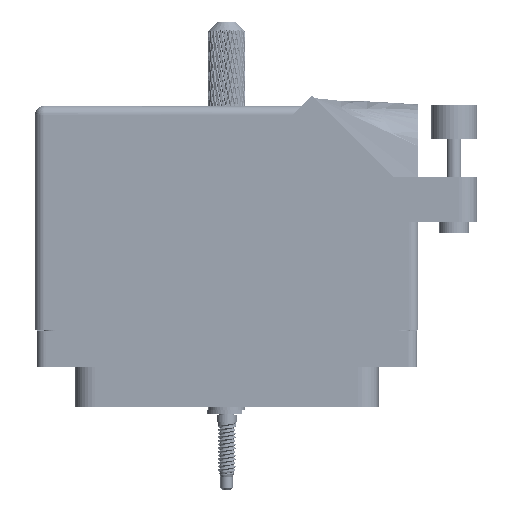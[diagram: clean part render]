
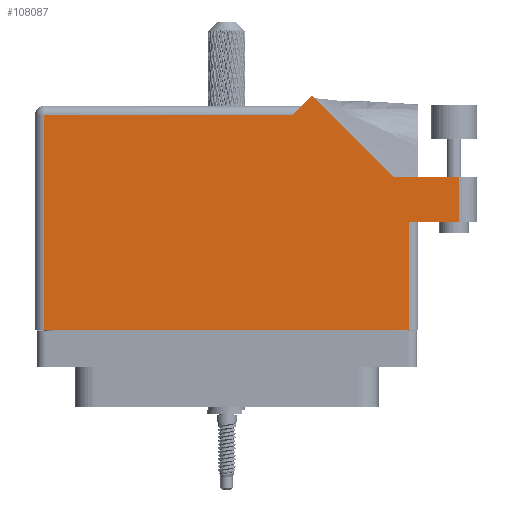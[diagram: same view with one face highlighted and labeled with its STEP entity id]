
A CAD part, front view. The second image highlights one B-rep face of the part: STEP entity #108087.
In plain terms, the highlighted face is planar.
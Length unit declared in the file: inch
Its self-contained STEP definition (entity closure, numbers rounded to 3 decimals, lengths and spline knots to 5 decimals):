
#319 = CARTESIAN_POINT ( 'NONE',  ( -1.306, 1.368, 0.455 ) ) ;
#4055 = ORIENTED_EDGE ( 'NONE', *, *, #53779, .T. ) ;
#4929 = DIRECTION ( 'NONE',  ( 0., 1., 0. ) ) ;
#6549 = ORIENTED_EDGE ( 'NONE', *, *, #40365, .T. ) ;
#8593 = VERTEX_POINT ( 'NONE', #75988 ) ;
#8964 = LINE ( 'NONE', #59721, #91401 ) ;
#10698 = VECTOR ( 'NONE', #41146, 39.37008 ) ;
#11083 = VERTEX_POINT ( 'NONE', #98812 ) ;
#12020 = ORIENTED_EDGE ( 'NONE', *, *, #70977, .T. ) ;
#14296 = LINE ( 'NONE', #103836, #85065 ) ;
#14906 = LINE ( 'NONE', #58714, #114394 ) ;
#15267 = DIRECTION ( 'NONE',  ( 0., -1., 0. ) ) ;
#15478 = VERTEX_POINT ( 'NONE', #91590 ) ;
#21665 = CARTESIAN_POINT ( 'NONE',  ( 1.14042, 0.944, 0.455 ) ) ;
#21743 = CARTESIAN_POINT ( 'NONE',  ( -1.306, 1.43, 0.455 ) ) ;
#21824 = LINE ( 'NONE', #57340, #115629 ) ;
#22697 = ORIENTED_EDGE ( 'NONE', *, *, #76236, .T. ) ;
#24972 = ORIENTED_EDGE ( 'NONE', *, *, #84708, .T. ) ;
#30084 = PLANE ( 'NONE',  #43974 ) ;
#38649 = CARTESIAN_POINT ( 'NONE',  ( 1.581, 0.637, 0.455 ) ) ;
#39071 = CARTESIAN_POINT ( 'NONE',  ( -1.244, 1.368, 0.455 ) ) ;
#39729 = VERTEX_POINT ( 'NONE', #39071 ) ;
#40365 = EDGE_CURVE ( 'NONE', #104644, #44992, #14296, .T. ) ;
#41146 = DIRECTION ( 'NONE',  ( 1., 0., 0. ) ) ;
#42696 = CARTESIAN_POINT ( 'NONE',  ( -1.244, -0.1, 0.455 ) ) ;
#43974 = AXIS2_PLACEMENT_3D ( 'NONE', #21743, #115491, #44368 ) ;
#44166 = EDGE_CURVE ( 'NONE', #70256, #11083, #14906, .T. ) ;
#44368 = DIRECTION ( 'NONE',  ( -1., 0., 0. ) ) ;
#44992 = VERTEX_POINT ( 'NONE', #54148 ) ;
#46527 = DIRECTION ( 'NONE',  ( -1., 0., 0. ) ) ;
#47803 = EDGE_CURVE ( 'NONE', #62975, #8593, #54138, .T. ) ;
#48067 = LINE ( 'NONE', #21665, #49534 ) ;
#49534 = VECTOR ( 'NONE', #67746, 39.37008 ) ;
#52033 = DIRECTION ( 'NONE',  ( 1., 0., 0. ) ) ;
#53217 = CARTESIAN_POINT ( 'NONE',  ( -1.306, -0.1, 0.455 ) ) ;
#53779 = EDGE_CURVE ( 'NONE', #71294, #104644, #93144, .T. ) ;
#54138 = LINE ( 'NONE', #53217, #66883 ) ;
#54148 = CARTESIAN_POINT ( 'NONE',  ( 1.581, 0.944, 0.455 ) ) ;
#57340 = CARTESIAN_POINT ( 'NONE',  ( 1.244, 0.637, 0.455 ) ) ;
#58046 = CARTESIAN_POINT ( 'NONE',  ( 1.244, 0.637, 0.455 ) ) ;
#58714 = CARTESIAN_POINT ( 'NONE',  ( 0.513, 1.43, 0.455 ) ) ;
#59201 = VECTOR ( 'NONE', #82179, 39.37008 ) ;
#59239 = ORIENTED_EDGE ( 'NONE', *, *, #117805, .T. ) ;
#59721 = CARTESIAN_POINT ( 'NONE',  ( -1.244, -0.1, 0.455 ) ) ;
#59876 = DIRECTION ( 'NONE',  ( -0.707, -0.707, 0. ) ) ;
#62975 = VERTEX_POINT ( 'NONE', #42696 ) ;
#66465 = DIRECTION ( 'NONE',  ( 0., 1., 0. ) ) ;
#66883 = VECTOR ( 'NONE', #52033, 39.37008 ) ;
#67746 = DIRECTION ( 'NONE',  ( -0.707, 0.707, 0. ) ) ;
#67803 = CARTESIAN_POINT ( 'NONE',  ( 1.306, 0.637, 0.455 ) ) ;
#70256 = VERTEX_POINT ( 'NONE', #93025 ) ;
#70977 = EDGE_CURVE ( 'NONE', #39729, #62975, #8964, .T. ) ;
#71212 = EDGE_LOOP ( 'NONE', ( #4055, #6549, #59239, #24972, #100927, #22697, #12020, #74295, #79947 ) ) ;
#71294 = VERTEX_POINT ( 'NONE', #58046 ) ;
#74295 = ORIENTED_EDGE ( 'NONE', *, *, #47803, .T. ) ;
#74373 = CARTESIAN_POINT ( 'NONE',  ( 1.706, 0.944, 0.455 ) ) ;
#75988 = CARTESIAN_POINT ( 'NONE',  ( 1.244, -0.1, 0.455 ) ) ;
#76236 = EDGE_CURVE ( 'NONE', #11083, #39729, #116098, .T. ) ;
#78447 = EDGE_CURVE ( 'NONE', #8593, #71294, #21824, .T. ) ;
#79597 = FACE_OUTER_BOUND ( 'NONE', #71212, .T. ) ;
#79947 = ORIENTED_EDGE ( 'NONE', *, *, #78447, .T. ) ;
#82179 = DIRECTION ( 'NONE',  ( -1., 0., 0. ) ) ;
#84708 = EDGE_CURVE ( 'NONE', #15478, #70256, #48067, .T. ) ;
#85065 = VECTOR ( 'NONE', #4929, 39.37008 ) ;
#86117 = VECTOR ( 'NONE', #46527, 39.37008 ) ;
#91401 = VECTOR ( 'NONE', #15267, 39.37008 ) ;
#91590 = CARTESIAN_POINT ( 'NONE',  ( 1.14042, 0.944, 0.455 ) ) ;
#93025 = CARTESIAN_POINT ( 'NONE',  ( 0.58371, 1.50071, 0.455 ) ) ;
#93144 = LINE ( 'NONE', #67803, #10698 ) ;
#98812 = CARTESIAN_POINT ( 'NONE',  ( 0.451, 1.368, 0.455 ) ) ;
#100927 = ORIENTED_EDGE ( 'NONE', *, *, #44166, .T. ) ;
#101546 = LINE ( 'NONE', #74373, #86117 ) ;
#103836 = CARTESIAN_POINT ( 'NONE',  ( 1.581, 0.944, 0.455 ) ) ;
#104644 = VERTEX_POINT ( 'NONE', #38649 ) ;
#108087 = ADVANCED_FACE ( 'NONE', ( #79597 ), #30084, .F. ) ;
#114394 = VECTOR ( 'NONE', #59876, 39.37008 ) ;
#115491 = DIRECTION ( 'NONE',  ( 0., 0., -1. ) ) ;
#115629 = VECTOR ( 'NONE', #66465, 39.37008 ) ;
#116098 = LINE ( 'NONE', #319, #59201 ) ;
#117805 = EDGE_CURVE ( 'NONE', #44992, #15478, #101546, .T. ) ;
